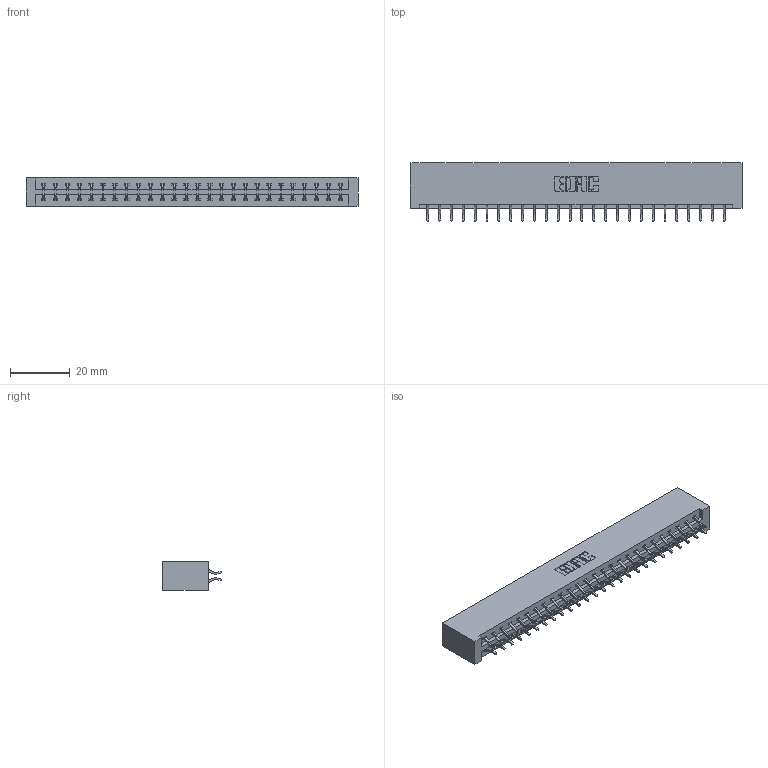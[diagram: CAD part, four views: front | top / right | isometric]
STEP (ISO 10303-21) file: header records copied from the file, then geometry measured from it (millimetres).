
FILE_DESCRIPTION (( 'STEP AP203' ), '1' );
FILE_NAME ('387-052-556-201.STEP', '2018-09-20T21:19:55', ( '' ), ( '' ), 'SwSTEP 2.0', 'SolidWorks 2016', '' );
FILE_SCHEMA (( 'CONFIG_CONTROL_DESIGN' ));
Length unit declared in the file: inch
Products named in the file (3): 337 Part_No Mounting Lugs; 345-292-001_556 Tail; 387-052-556-201
Assembly tree (53 placements, depth 2):
  387-052-556-201
    337 Part_No Mounting Lugs
    345-292-001_556 Tail  x52
Bounding box: 110.9 x 19.57 x 9.4 mm (x, y, z)
Volume: 12232.8 mm3; surface area: 13675.1 mm2
Topology: 53 solids, 53 shells, 3226 faces, 9595 edges, 6326 vertices
Faces by surface type: plane 2250, cylinder 976
Entity records: 22171 total; most frequent: CARTESIAN_POINT 3762, ORIENTED_EDGE 3686, DIRECTION 3211, EDGE_CURVE 1843, LINE 1715, VECTOR 1715, VERTEX_POINT 1226, AXIS2_PLACEMENT_3D 748
